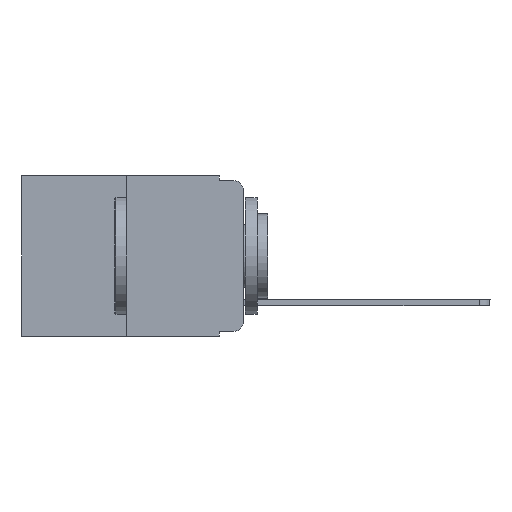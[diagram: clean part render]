
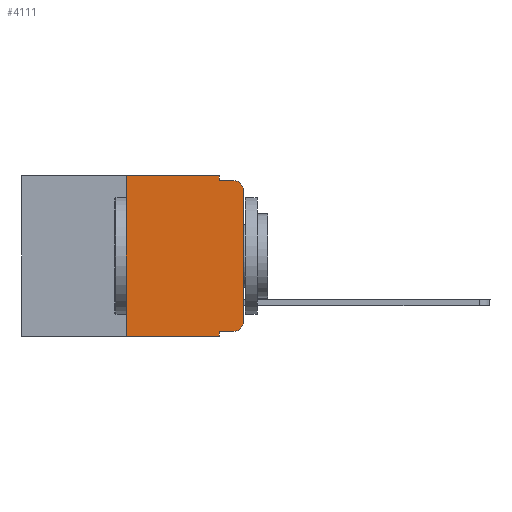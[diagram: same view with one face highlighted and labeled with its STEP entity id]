
A CAD part, left-side view. The second image highlights one B-rep face of the part: STEP entity #4111.
In plain terms, the highlighted planar face has unit normal (-1, 0, 0).
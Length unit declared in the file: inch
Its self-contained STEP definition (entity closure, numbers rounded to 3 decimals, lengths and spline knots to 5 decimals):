
#93 = VERTEX_POINT ( 'NONE', #6496 ) ;
#177 = DIRECTION ( 'NONE',  ( 0., 0., -1. ) ) ;
#244 = CARTESIAN_POINT ( 'NONE',  ( 0., 0.051, 0. ) ) ;
#542 = DIRECTION ( 'NONE',  ( 0., 0., -1. ) ) ;
#878 = DIRECTION ( 'NONE',  ( 0., 0., -1. ) ) ;
#1318 = AXIS2_PLACEMENT_3D ( 'NONE', #13437, #6151, #177 ) ;
#1433 = LINE ( 'NONE', #16486, #18849 ) ;
#1887 = CARTESIAN_POINT ( 'NONE',  ( 0., 0.051, -0.333 ) ) ;
#2112 = VECTOR ( 'NONE', #15162, 39.37008 ) ;
#2265 = LINE ( 'NONE', #17616, #17404 ) ;
#2731 = CARTESIAN_POINT ( 'NONE',  ( 0., 0.473, -0.343 ) ) ;
#2798 = VERTEX_POINT ( 'NONE', #4307 ) ;
#3040 = EDGE_LOOP ( 'NONE', ( #17916, #10084, #18697, #5525, #13492, #15044, #6756, #3635, #9213, #18081 ) ) ;
#3078 = LINE ( 'NONE', #244, #15968 ) ;
#3587 = CARTESIAN_POINT ( 'NONE',  ( 0., 0.02, -0.01 ) ) ;
#3635 = ORIENTED_EDGE ( 'NONE', *, *, #16106, .F. ) ;
#4086 = LINE ( 'NONE', #8239, #13320 ) ;
#4111 = ADVANCED_FACE ( 'NONE', ( #4629 ), #16635, .F. ) ;
#4307 = CARTESIAN_POINT ( 'NONE',  ( 0., 0.051, 0. ) ) ;
#4629 = FACE_OUTER_BOUND ( 'NONE', #3040, .T. ) ;
#4917 = LINE ( 'NONE', #9723, #15061 ) ;
#5321 = EDGE_CURVE ( 'NONE', #17198, #9184, #18293, .T. ) ;
#5357 = VERTEX_POINT ( 'NONE', #10465 ) ;
#5372 = EDGE_CURVE ( 'NONE', #5357, #9948, #1433, .T. ) ;
#5525 = ORIENTED_EDGE ( 'NONE', *, *, #7129, .F. ) ;
#5785 = CARTESIAN_POINT ( 'NONE',  ( 0., 0.051, 0. ) ) ;
#5873 = VECTOR ( 'NONE', #878, 39.37008 ) ;
#6151 = DIRECTION ( 'NONE',  ( -1., 0., 0. ) ) ;
#6352 = CIRCLE ( 'NONE', #15769, 0.02 ) ;
#6428 = DIRECTION ( 'NONE',  ( 0., 0., -1. ) ) ;
#6496 = CARTESIAN_POINT ( 'NONE',  ( 0., 0.051, -0.333 ) ) ;
#6515 = CARTESIAN_POINT ( 'NONE',  ( 0., 0., -0.313 ) ) ;
#6666 = DIRECTION ( 'NONE',  ( 0., -1., 0. ) ) ;
#6756 = ORIENTED_EDGE ( 'NONE', *, *, #16228, .T. ) ;
#7129 = EDGE_CURVE ( 'NONE', #2798, #9065, #3078, .T. ) ;
#7679 = DIRECTION ( 'NONE',  ( 1., 0., 0. ) ) ;
#7721 = EDGE_CURVE ( 'NONE', #9948, #2798, #4917, .T. ) ;
#8239 = CARTESIAN_POINT ( 'NONE',  ( 0., 0.051, -0.01 ) ) ;
#9065 = VERTEX_POINT ( 'NONE', #16207 ) ;
#9154 = CARTESIAN_POINT ( 'NONE',  ( 0., 0.473, 0. ) ) ;
#9184 = VERTEX_POINT ( 'NONE', #3587 ) ;
#9213 = ORIENTED_EDGE ( 'NONE', *, *, #15778, .T. ) ;
#9723 = CARTESIAN_POINT ( 'NONE',  ( 0., 0.473, 0. ) ) ;
#9948 = VERTEX_POINT ( 'NONE', #13189 ) ;
#10084 = ORIENTED_EDGE ( 'NONE', *, *, #5321, .T. ) ;
#10394 = DIRECTION ( 'NONE',  ( 0., -1., 0. ) ) ;
#10465 = CARTESIAN_POINT ( 'NONE',  ( 0., 0.25, -0.343 ) ) ;
#10584 = VECTOR ( 'NONE', #10394, 39.37008 ) ;
#10665 = DIRECTION ( 'NONE',  ( 0., 0., 1. ) ) ;
#10941 = DIRECTION ( 'NONE',  ( -1., 0., 0. ) ) ;
#11140 = CARTESIAN_POINT ( 'NONE',  ( 0., 0., -0.03 ) ) ;
#11203 = DIRECTION ( 'NONE',  ( 0., -1., 0. ) ) ;
#11809 = EDGE_CURVE ( 'NONE', #9065, #9184, #4086, .T. ) ;
#12968 = VERTEX_POINT ( 'NONE', #6515 ) ;
#12991 = DIRECTION ( 'NONE',  ( 0., 0., 1. ) ) ;
#13189 = CARTESIAN_POINT ( 'NONE',  ( 0., 0.25, 0. ) ) ;
#13320 = VECTOR ( 'NONE', #6666, 39.37008 ) ;
#13369 = CARTESIAN_POINT ( 'NONE',  ( 0., 0.02, -0.333 ) ) ;
#13437 = CARTESIAN_POINT ( 'NONE',  ( 0., 0.02, -0.03 ) ) ;
#13492 = ORIENTED_EDGE ( 'NONE', *, *, #7721, .F. ) ;
#13684 = DIRECTION ( 'NONE',  ( 0., 0., -1. ) ) ;
#13689 = LINE ( 'NONE', #1887, #2112 ) ;
#14200 = CARTESIAN_POINT ( 'NONE',  ( 0., 0.02, -0.313 ) ) ;
#14784 = VERTEX_POINT ( 'NONE', #15355 ) ;
#15044 = ORIENTED_EDGE ( 'NONE', *, *, #5372, .F. ) ;
#15061 = VECTOR ( 'NONE', #11203, 39.37008 ) ;
#15162 = DIRECTION ( 'NONE',  ( 0., -1., 0. ) ) ;
#15355 = CARTESIAN_POINT ( 'NONE',  ( 0., 0.051, -0.343 ) ) ;
#15769 = AXIS2_PLACEMENT_3D ( 'NONE', #14200, #10941, #542 ) ;
#15778 = EDGE_CURVE ( 'NONE', #93, #16246, #13689, .T. ) ;
#15968 = VECTOR ( 'NONE', #6428, 39.37008 ) ;
#16084 = AXIS2_PLACEMENT_3D ( 'NONE', #9154, #7679, #13684 ) ;
#16106 = EDGE_CURVE ( 'NONE', #93, #14784, #19270, .T. ) ;
#16207 = CARTESIAN_POINT ( 'NONE',  ( 0., 0.051, -0.01 ) ) ;
#16214 = LINE ( 'NONE', #2731, #10584 ) ;
#16228 = EDGE_CURVE ( 'NONE', #5357, #14784, #16214, .T. ) ;
#16246 = VERTEX_POINT ( 'NONE', #13369 ) ;
#16486 = CARTESIAN_POINT ( 'NONE',  ( 0., 0.25, 0. ) ) ;
#16635 = PLANE ( 'NONE',  #16084 ) ;
#17130 = EDGE_CURVE ( 'NONE', #16246, #12968, #6352, .T. ) ;
#17198 = VERTEX_POINT ( 'NONE', #11140 ) ;
#17404 = VECTOR ( 'NONE', #12991, 39.37008 ) ;
#17616 = CARTESIAN_POINT ( 'NONE',  ( 0., 0., 0. ) ) ;
#17916 = ORIENTED_EDGE ( 'NONE', *, *, #18874, .T. ) ;
#18081 = ORIENTED_EDGE ( 'NONE', *, *, #17130, .T. ) ;
#18293 = CIRCLE ( 'NONE', #1318, 0.02 ) ;
#18697 = ORIENTED_EDGE ( 'NONE', *, *, #11809, .F. ) ;
#18849 = VECTOR ( 'NONE', #10665, 39.37008 ) ;
#18874 = EDGE_CURVE ( 'NONE', #12968, #17198, #2265, .T. ) ;
#19270 = LINE ( 'NONE', #5785, #5873 ) ;
